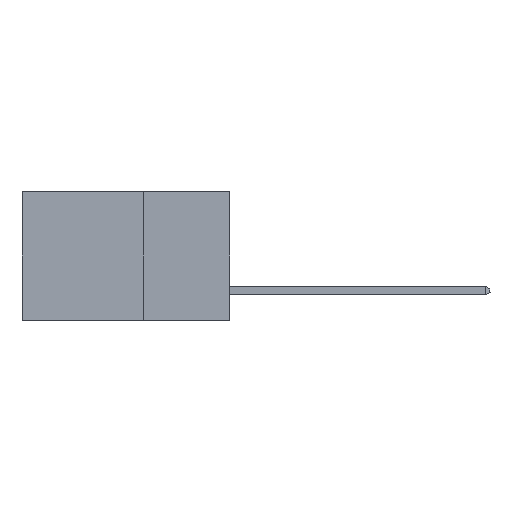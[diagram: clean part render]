
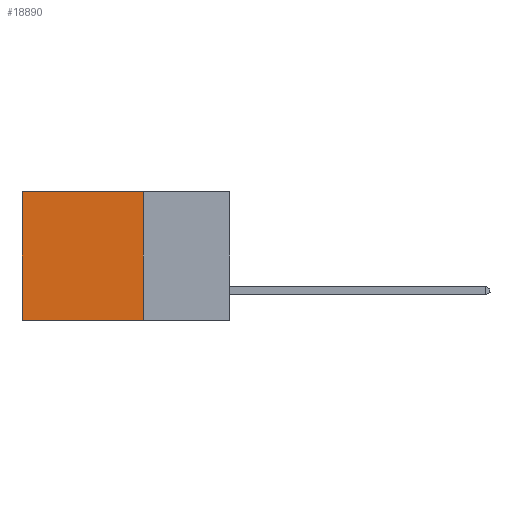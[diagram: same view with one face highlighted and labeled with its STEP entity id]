
A CAD part, left-side view. The second image highlights one B-rep face of the part: STEP entity #18890.
In plain terms, the highlighted planar face has unit normal (-1, 0, 0).
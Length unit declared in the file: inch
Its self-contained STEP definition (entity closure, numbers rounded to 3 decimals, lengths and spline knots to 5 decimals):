
#95 = VERTEX_POINT ( 'NONE', #12861 ) ;
#1147 = ORIENTED_EDGE ( 'NONE', *, *, #11013, .T. ) ;
#2541 = LINE ( 'NONE', #25364, #20682 ) ;
#3610 = CARTESIAN_POINT ( 'NONE',  ( 0.298, 0.25, 0. ) ) ;
#5192 = ORIENTED_EDGE ( 'NONE', *, *, #13547, .F. ) ;
#5711 = CARTESIAN_POINT ( 'NONE',  ( 0.298, 0.6, 0. ) ) ;
#5800 = VERTEX_POINT ( 'NONE', #3610 ) ;
#5879 = DIRECTION ( 'NONE',  ( 0., 0., -1. ) ) ;
#6103 = VECTOR ( 'NONE', #22564, 39.37008 ) ;
#8284 = CARTESIAN_POINT ( 'NONE',  ( 0.298, 0.25, -0.37 ) ) ;
#8708 = LINE ( 'NONE', #20057, #20529 ) ;
#8791 = EDGE_LOOP ( 'NONE', ( #1147, #21507, #5192, #13485 ) ) ;
#9108 = CARTESIAN_POINT ( 'NONE',  ( 0.298, 0.6, -0.37 ) ) ;
#10645 = DIRECTION ( 'NONE',  ( 1., 0., 0. ) ) ;
#10690 = VECTOR ( 'NONE', #15855, 39.37008 ) ;
#11013 = EDGE_CURVE ( 'NONE', #23264, #21726, #2541, .T. ) ;
#12861 = CARTESIAN_POINT ( 'NONE',  ( 0.298, 0.25, -0.37 ) ) ;
#13485 = ORIENTED_EDGE ( 'NONE', *, *, #17450, .T. ) ;
#13519 = EDGE_CURVE ( 'NONE', #95, #21726, #30494, .T. ) ;
#13547 = EDGE_CURVE ( 'NONE', #5800, #95, #8708, .T. ) ;
#15708 = FACE_OUTER_BOUND ( 'NONE', #8791, .T. ) ;
#15855 = DIRECTION ( 'NONE',  ( 0., 1., 0. ) ) ;
#16160 = CARTESIAN_POINT ( 'NONE',  ( 0.298, 0.25, 0. ) ) ;
#17450 = EDGE_CURVE ( 'NONE', #5800, #23264, #18818, .T. ) ;
#17656 = CARTESIAN_POINT ( 'NONE',  ( 0.298, 0.25, 0. ) ) ;
#18818 = LINE ( 'NONE', #16160, #10690 ) ;
#18890 = ADVANCED_FACE ( 'NONE', ( #15708 ), #27284, .F. ) ;
#20038 = DIRECTION ( 'NONE',  ( 0., 0., -1. ) ) ;
#20057 = CARTESIAN_POINT ( 'NONE',  ( 0.298, 0.25, 0. ) ) ;
#20529 = VECTOR ( 'NONE', #5879, 39.37008 ) ;
#20682 = VECTOR ( 'NONE', #20866, 39.37008 ) ;
#20866 = DIRECTION ( 'NONE',  ( 0., 0., -1. ) ) ;
#21507 = ORIENTED_EDGE ( 'NONE', *, *, #13519, .F. ) ;
#21726 = VERTEX_POINT ( 'NONE', #9108 ) ;
#22564 = DIRECTION ( 'NONE',  ( 0., 1., 0. ) ) ;
#23264 = VERTEX_POINT ( 'NONE', #5711 ) ;
#25364 = CARTESIAN_POINT ( 'NONE',  ( 0.298, 0.6, 0. ) ) ;
#27284 = PLANE ( 'NONE',  #30031 ) ;
#30031 = AXIS2_PLACEMENT_3D ( 'NONE', #17656, #10645, #20038 ) ;
#30494 = LINE ( 'NONE', #8284, #6103 ) ;
